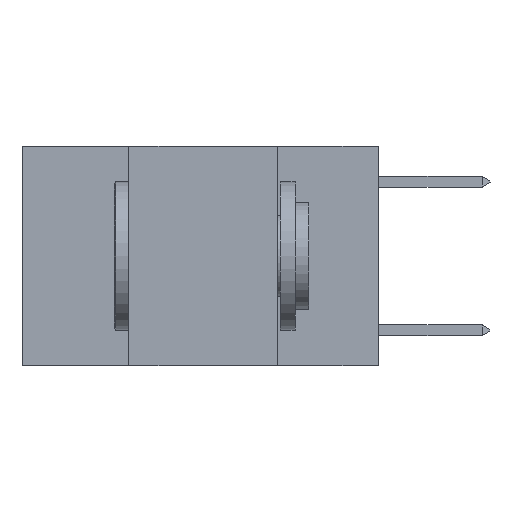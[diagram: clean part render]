
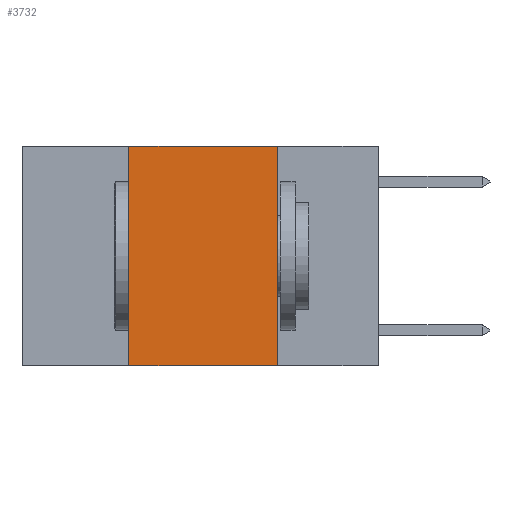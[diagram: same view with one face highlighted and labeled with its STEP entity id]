
A CAD part, left-side view. The second image highlights one B-rep face of the part: STEP entity #3732.
In plain terms, the highlighted planar face has unit normal (-1, 0, 0).
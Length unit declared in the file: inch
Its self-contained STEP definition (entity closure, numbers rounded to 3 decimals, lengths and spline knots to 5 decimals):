
#555 = VECTOR ( 'NONE', #13047, 39.37008 ) ;
#1233 = DIRECTION ( 'NONE',  ( 0., -1., 0. ) ) ;
#1402 = VERTEX_POINT ( 'NONE', #6132 ) ;
#1699 = VERTEX_POINT ( 'NONE', #13228 ) ;
#1972 = ORIENTED_EDGE ( 'NONE', *, *, #2587, .T. ) ;
#2587 = EDGE_CURVE ( 'NONE', #1402, #14401, #10755, .T. ) ;
#2762 = DIRECTION ( 'NONE',  ( 0., 0., -1. ) ) ;
#2812 = LINE ( 'NONE', #8890, #555 ) ;
#2849 = DIRECTION ( 'NONE',  ( 0., -1., 0. ) ) ;
#3732 = ADVANCED_FACE ( 'NONE', ( #3910 ), #8024, .F. ) ;
#3831 = EDGE_CURVE ( 'NONE', #1699, #14401, #2812, .T. ) ;
#3910 = FACE_OUTER_BOUND ( 'NONE', #5260, .T. ) ;
#4858 = EDGE_CURVE ( 'NONE', #7607, #1699, #9735, .T. ) ;
#5260 = EDGE_LOOP ( 'NONE', ( #8977, #6417, #9656, #1972 ) ) ;
#5435 = VECTOR ( 'NONE', #2849, 39.37008 ) ;
#6132 = CARTESIAN_POINT ( 'NONE',  ( 0., 0.42, -0.37 ) ) ;
#6417 = ORIENTED_EDGE ( 'NONE', *, *, #4858, .F. ) ;
#7006 = CARTESIAN_POINT ( 'NONE',  ( 0., 0.6, -0.37 ) ) ;
#7566 = CARTESIAN_POINT ( 'NONE',  ( 0., 0.17, -0.37 ) ) ;
#7607 = VERTEX_POINT ( 'NONE', #10132 ) ;
#8024 = PLANE ( 'NONE',  #10756 ) ;
#8141 = CARTESIAN_POINT ( 'NONE',  ( 0., 0.42, 0. ) ) ;
#8167 = EDGE_CURVE ( 'NONE', #1402, #7607, #14704, .T. ) ;
#8780 = CARTESIAN_POINT ( 'NONE',  ( 0., 0.6, 0. ) ) ;
#8890 = CARTESIAN_POINT ( 'NONE',  ( 0., 0.17, 0. ) ) ;
#8977 = ORIENTED_EDGE ( 'NONE', *, *, #3831, .F. ) ;
#9263 = DIRECTION ( 'NONE',  ( 0., 0., 1. ) ) ;
#9656 = ORIENTED_EDGE ( 'NONE', *, *, #8167, .F. ) ;
#9680 = VECTOR ( 'NONE', #1233, 39.37008 ) ;
#9735 = LINE ( 'NONE', #12018, #9680 ) ;
#10132 = CARTESIAN_POINT ( 'NONE',  ( 0., 0.42, 0. ) ) ;
#10755 = LINE ( 'NONE', #7006, #5435 ) ;
#10756 = AXIS2_PLACEMENT_3D ( 'NONE', #8780, #11222, #2762 ) ;
#11222 = DIRECTION ( 'NONE',  ( 1., 0., 0. ) ) ;
#12018 = CARTESIAN_POINT ( 'NONE',  ( 0., 0.6, 0. ) ) ;
#13047 = DIRECTION ( 'NONE',  ( 0., 0., -1. ) ) ;
#13228 = CARTESIAN_POINT ( 'NONE',  ( 0., 0.17, 0. ) ) ;
#14401 = VERTEX_POINT ( 'NONE', #7566 ) ;
#14621 = VECTOR ( 'NONE', #9263, 39.37008 ) ;
#14704 = LINE ( 'NONE', #8141, #14621 ) ;
